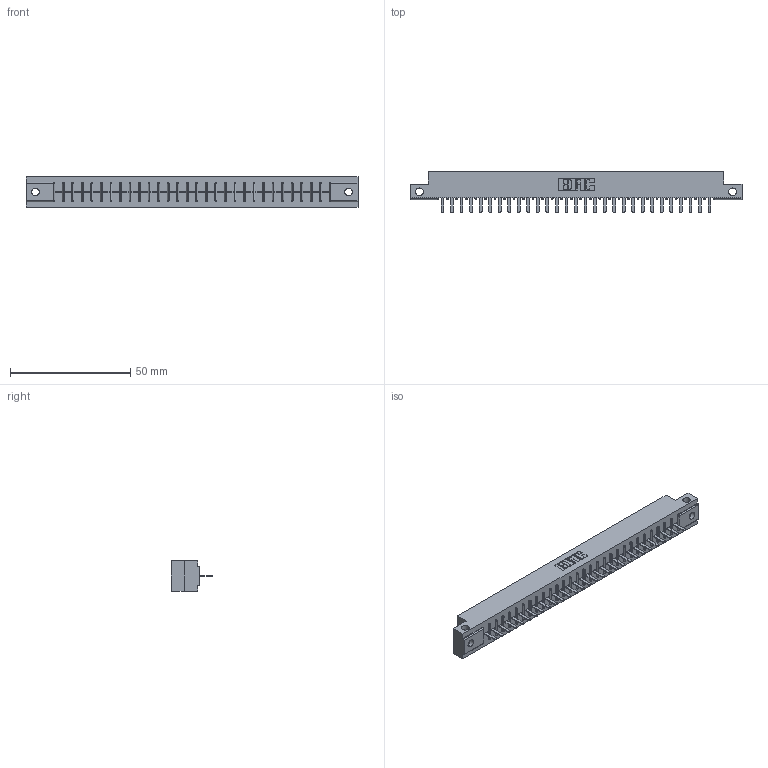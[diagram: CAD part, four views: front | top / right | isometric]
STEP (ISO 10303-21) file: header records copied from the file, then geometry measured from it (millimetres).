
FILE_DESCRIPTION (( 'STEP AP203' ), '1' );
FILE_NAME ('356-029-420-112.STEP', '2020-09-23T19:03:32', ( '' ), ( '' ), 'SwSTEP 2.0', 'SolidWorks 2020', '' );
FILE_SCHEMA (( 'CONFIG_CONTROL_DESIGN' ));
Length unit declared in the file: inch
Products named in the file (3): 306-290-001_120; 356-029-420-112; 306 Part_.128 Dia
Assembly tree (30 placements, depth 2):
  356-029-420-112
    306 Part_.128 Dia
    306-290-001_120  x29
Bounding box: 137.92 x 17.12 x 12.7 mm (x, y, z)
Volume: 14933.3 mm3; surface area: 15238.5 mm2
Topology: 30 solids, 30 shells, 2158 faces, 6065 edges, 3882 vertices
Faces by surface type: plane 1431, cylinder 611, sphere 116
Entity records: 29090 total; most frequent: CARTESIAN_POINT 4930, ORIENTED_EDGE 4842, DIRECTION 4801, EDGE_CURVE 2421, VECTOR 1871, LINE 1871, VERTEX_POINT 1530, AXIS2_PLACEMENT_3D 1465
